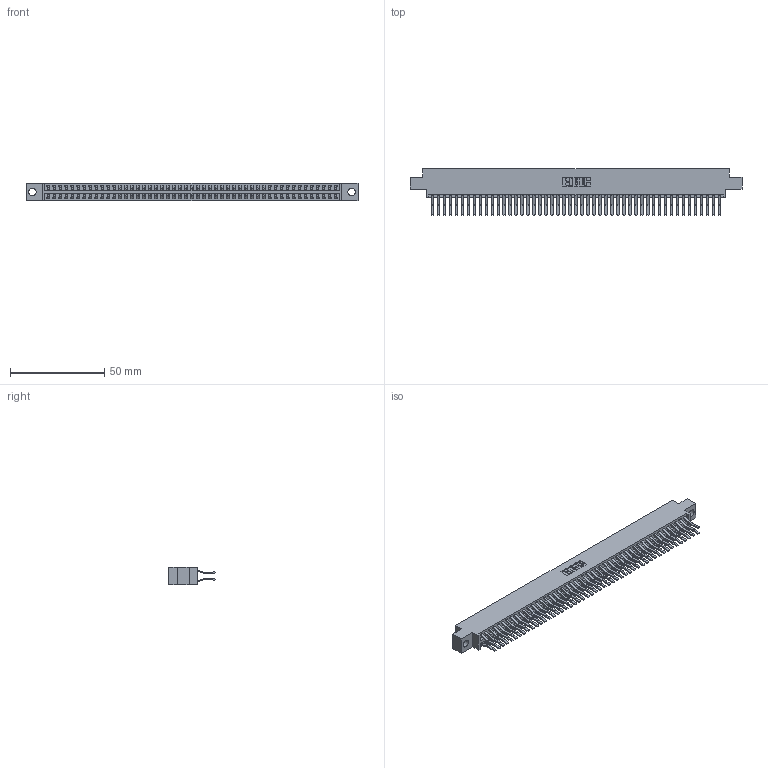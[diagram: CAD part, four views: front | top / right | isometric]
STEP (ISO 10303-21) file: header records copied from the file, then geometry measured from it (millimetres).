
FILE_DESCRIPTION (( 'STEP AP203' ), '1' );
FILE_NAME ('346-098-560-804.STEP', '2022-05-26T19:31:02', ( '' ), ( '' ), 'SwSTEP 2.0', 'SolidWorks 2020', '' );
FILE_SCHEMA (( 'CONFIG_CONTROL_DESIGN' ));
Length unit declared in the file: inch
Products named in the file (3): 346-098-560-804; 345-292-001_560 Tail; 346 Part_0.170 Offset - 0.156 Dia-TH
Assembly tree (99 placements, depth 2):
  346-098-560-804
    346 Part_0.170 Offset - 0.156 Dia-TH
    345-292-001_560 Tail  x98
Bounding box: 176.15 x 24.78 x 9.4 mm (x, y, z)
Volume: 17612.9 mm3; surface area: 26061.4 mm2
Topology: 99 solids, 99 shells, 5432 faces, 16155 edges, 10638 vertices
Faces by surface type: plane 3524, cylinder 1908
Entity records: 31675 total; most frequent: CARTESIAN_POINT 5218, ORIENTED_EDGE 5150, DIRECTION 4651, EDGE_CURVE 2575, VECTOR 2243, LINE 2243, VERTEX_POINT 1714, AXIS2_PLACEMENT_3D 1204
